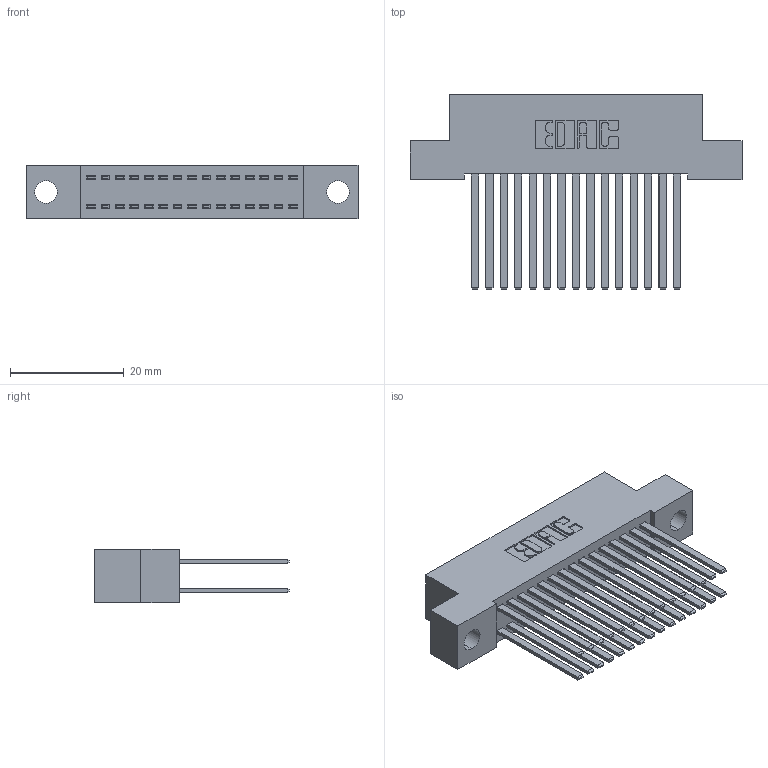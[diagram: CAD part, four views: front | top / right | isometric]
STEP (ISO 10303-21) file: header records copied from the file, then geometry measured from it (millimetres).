
FILE_DESCRIPTION (( 'STEP AP203' ), '1' );
FILE_NAME ('342-030-544-204.STEP', '2018-08-11T15:44:00', ( '' ), ( '' ), 'SwSTEP 2.0', 'SolidWorks 2016', '' );
FILE_SCHEMA (( 'CONFIG_CONTROL_DESIGN' ));
Length unit declared in the file: inch
Products named in the file (3): 342 Part_.156 TH; 345-292-001_345-293-144; 342-030-544-204
Assembly tree (31 placements, depth 2):
  342-030-544-204
    342 Part_.156 TH
    345-292-001_345-293-144  x30
Bounding box: 58.42 x 34.3 x 9.4 mm (x, y, z)
Volume: 5454.8 mm3; surface area: 9202.5 mm2
Topology: 31 solids, 31 shells, 1490 faces, 4409 edges, 2898 vertices
Faces by surface type: plane 1026, cylinder 464
Entity records: 12829 total; most frequent: CARTESIAN_POINT 2154, ORIENTED_EDGE 2090, DIRECTION 1885, EDGE_CURVE 1045, LINE 921, VECTOR 921, VERTEX_POINT 694, AXIS2_PLACEMENT_3D 482
